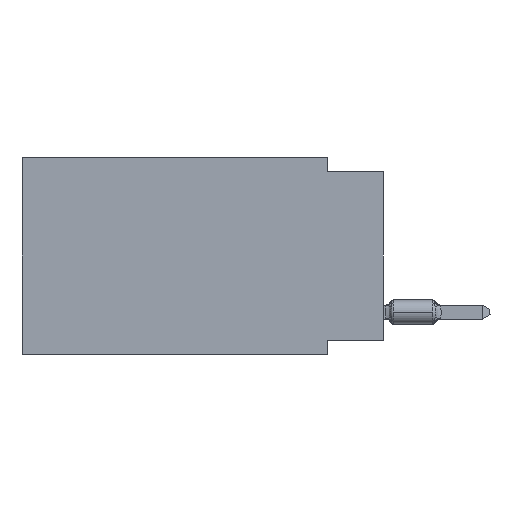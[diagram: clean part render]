
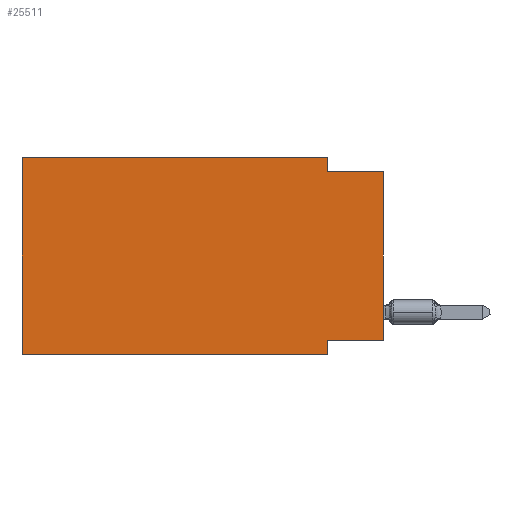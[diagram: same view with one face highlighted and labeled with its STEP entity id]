
A CAD part, left-side view. The second image highlights one B-rep face of the part: STEP entity #25511.
In plain terms, the highlighted planar face has unit normal (-1, 0, 0).
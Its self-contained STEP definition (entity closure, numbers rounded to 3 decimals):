
#211 = VECTOR ( 'NONE', #15969, 1000. ) ;
#737 = CARTESIAN_POINT ( 'NONE',  ( 0., 0., -8.255 ) ) ;
#1993 = LINE ( 'NONE', #14495, #28546 ) ;
#3195 = CARTESIAN_POINT ( 'NONE',  ( 0., 16.383, -8.89 ) ) ;
#3349 = ORIENTED_EDGE ( 'NONE', *, *, #38278, .T. ) ;
#3760 = CARTESIAN_POINT ( 'NONE',  ( 0., 2.54, 0. ) ) ;
#6062 = VECTOR ( 'NONE', #16748, 1000. ) ;
#6255 = VERTEX_POINT ( 'NONE', #36869 ) ;
#6265 = DIRECTION ( 'NONE',  ( 0., -1., 0. ) ) ;
#6315 = VECTOR ( 'NONE', #9994, 1000. ) ;
#6390 = EDGE_CURVE ( 'NONE', #15019, #40174, #31111, .T. ) ;
#6506 = LINE ( 'NONE', #31550, #6315 ) ;
#6543 = LINE ( 'NONE', #37929, #211 ) ;
#7038 = VECTOR ( 'NONE', #22850, 1000. ) ;
#8182 = CARTESIAN_POINT ( 'NONE',  ( 0., 16.383, 0. ) ) ;
#8855 = ORIENTED_EDGE ( 'NONE', *, *, #33657, .F. ) ;
#9672 = VECTOR ( 'NONE', #19777, 1000. ) ;
#9879 = AXIS2_PLACEMENT_3D ( 'NONE', #8182, #26872, #30766 ) ;
#9994 = DIRECTION ( 'NONE',  ( 0., 0., 1. ) ) ;
#10680 = ORIENTED_EDGE ( 'NONE', *, *, #40117, .F. ) ;
#11426 = DIRECTION ( 'NONE',  ( 0., 0., 1. ) ) ;
#11946 = CARTESIAN_POINT ( 'NONE',  ( 0., 0., -0.635 ) ) ;
#12040 = ORIENTED_EDGE ( 'NONE', *, *, #27512, .F. ) ;
#12091 = FACE_OUTER_BOUND ( 'NONE', #15372, .T. ) ;
#12454 = DIRECTION ( 'NONE',  ( 0., 1., 0. ) ) ;
#13880 = CARTESIAN_POINT ( 'NONE',  ( 0., 0., -0.635 ) ) ;
#14495 = CARTESIAN_POINT ( 'NONE',  ( 0., 0., 0. ) ) ;
#14519 = LINE ( 'NONE', #40567, #30509 ) ;
#15019 = VERTEX_POINT ( 'NONE', #36330 ) ;
#15372 = EDGE_LOOP ( 'NONE', ( #3349, #12040, #8855, #10680, #27162, #25470, #40521, #34257 ) ) ;
#15969 = DIRECTION ( 'NONE',  ( 0., 0., -1. ) ) ;
#16003 = CARTESIAN_POINT ( 'NONE',  ( 0., 2.54, 0. ) ) ;
#16748 = DIRECTION ( 'NONE',  ( 0., -1., 0. ) ) ;
#16921 = VERTEX_POINT ( 'NONE', #19745 ) ;
#17227 = EDGE_CURVE ( 'NONE', #38528, #27879, #14519, .T. ) ;
#18537 = EDGE_CURVE ( 'NONE', #15019, #6255, #6506, .T. ) ;
#19745 = CARTESIAN_POINT ( 'NONE',  ( 0., 2.54, -0.635 ) ) ;
#19777 = DIRECTION ( 'NONE',  ( 0., 0., -1. ) ) ;
#19948 = EDGE_CURVE ( 'NONE', #27879, #40174, #6543, .T. ) ;
#22850 = DIRECTION ( 'NONE',  ( 0., -1., 0. ) ) ;
#25470 = ORIENTED_EDGE ( 'NONE', *, *, #6390, .T. ) ;
#25511 = ADVANCED_FACE ( 'NONE', ( #12091 ), #27691, .F. ) ;
#26872 = DIRECTION ( 'NONE',  ( 1., 0., 0. ) ) ;
#27162 = ORIENTED_EDGE ( 'NONE', *, *, #18537, .F. ) ;
#27512 = EDGE_CURVE ( 'NONE', #16921, #28818, #29696, .T. ) ;
#27691 = PLANE ( 'NONE',  #9879 ) ;
#27879 = VERTEX_POINT ( 'NONE', #35377 ) ;
#28546 = VECTOR ( 'NONE', #11426, 1000. ) ;
#28818 = VERTEX_POINT ( 'NONE', #11946 ) ;
#29035 = CARTESIAN_POINT ( 'NONE',  ( 0., 16.383, 0. ) ) ;
#29645 = CARTESIAN_POINT ( 'NONE',  ( 0., 2.54, -8.89 ) ) ;
#29696 = LINE ( 'NONE', #13880, #6062 ) ;
#30509 = VECTOR ( 'NONE', #12454, 1000. ) ;
#30766 = DIRECTION ( 'NONE',  ( 0., 0., -1. ) ) ;
#31111 = LINE ( 'NONE', #3195, #35978 ) ;
#31550 = CARTESIAN_POINT ( 'NONE',  ( 0., 16.383, 0. ) ) ;
#31877 = LINE ( 'NONE', #3760, #9672 ) ;
#32301 = LINE ( 'NONE', #29035, #7038 ) ;
#33657 = EDGE_CURVE ( 'NONE', #39386, #16921, #31877, .T. ) ;
#34257 = ORIENTED_EDGE ( 'NONE', *, *, #17227, .F. ) ;
#35377 = CARTESIAN_POINT ( 'NONE',  ( 0., 2.54, -8.255 ) ) ;
#35978 = VECTOR ( 'NONE', #6265, 1000. ) ;
#36330 = CARTESIAN_POINT ( 'NONE',  ( 0., 16.383, -8.89 ) ) ;
#36869 = CARTESIAN_POINT ( 'NONE',  ( 0., 16.383, 0. ) ) ;
#37929 = CARTESIAN_POINT ( 'NONE',  ( 0., 2.54, -8.89 ) ) ;
#38278 = EDGE_CURVE ( 'NONE', #38528, #28818, #1993, .T. ) ;
#38528 = VERTEX_POINT ( 'NONE', #737 ) ;
#39386 = VERTEX_POINT ( 'NONE', #16003 ) ;
#40117 = EDGE_CURVE ( 'NONE', #6255, #39386, #32301, .T. ) ;
#40174 = VERTEX_POINT ( 'NONE', #29645 ) ;
#40521 = ORIENTED_EDGE ( 'NONE', *, *, #19948, .F. ) ;
#40567 = CARTESIAN_POINT ( 'NONE',  ( 0., 0., -8.255 ) ) ;
